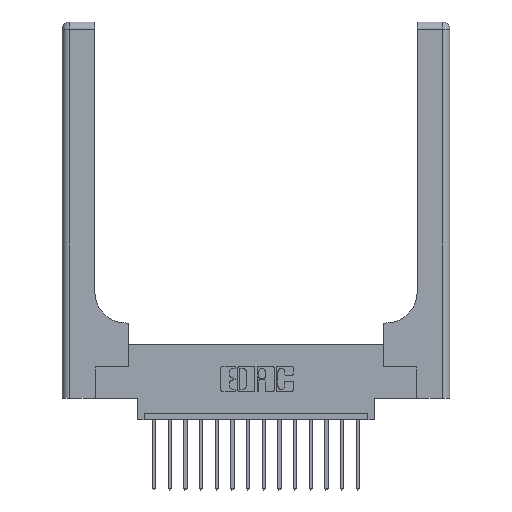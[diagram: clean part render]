
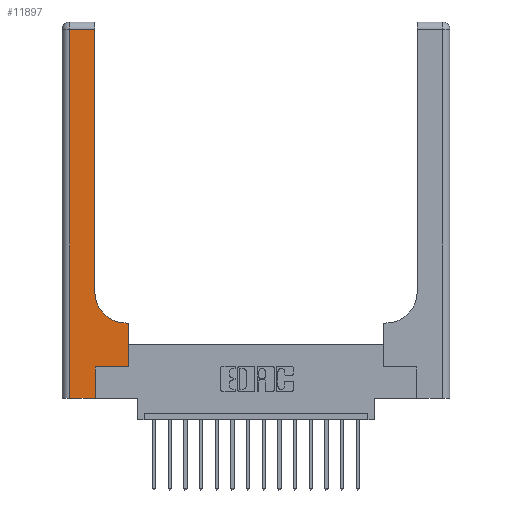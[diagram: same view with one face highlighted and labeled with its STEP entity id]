
A CAD part, top view. The second image highlights one B-rep face of the part: STEP entity #11897.
In plain terms, the highlighted planar face has unit normal (0, 0, 1).
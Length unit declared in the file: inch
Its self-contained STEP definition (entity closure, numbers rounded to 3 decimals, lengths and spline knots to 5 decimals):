
#103 = EDGE_CURVE ( 'NONE', #12529, #12269, #13879, .T. ) ;
#304 = EDGE_CURVE ( 'NONE', #2396, #16840, #3853, .T. ) ;
#818 = EDGE_CURVE ( 'NONE', #12269, #13218, #6470, .T. ) ;
#1005 = ORIENTED_EDGE ( 'NONE', *, *, #304, .T. ) ;
#1039 = DIRECTION ( 'NONE',  ( 1., 0., 0. ) ) ;
#1226 = EDGE_CURVE ( 'NONE', #9002, #12529, #13136, .T. ) ;
#1478 = DIRECTION ( 'NONE',  ( -1., 0., 0. ) ) ;
#1930 = CARTESIAN_POINT ( 'NONE',  ( 0.26, 0.85, 0.37 ) ) ;
#2396 = VERTEX_POINT ( 'NONE', #14128 ) ;
#2476 = VECTOR ( 'NONE', #17531, 39.37008 ) ;
#2568 = EDGE_CURVE ( 'NONE', #16840, #5805, #7296, .T. ) ;
#3481 = ORIENTED_EDGE ( 'NONE', *, *, #103, .T. ) ;
#3629 = CARTESIAN_POINT ( 'NONE',  ( 0.51, 0.85, 0.37 ) ) ;
#3701 = LINE ( 'NONE', #14926, #17962 ) ;
#3853 = CIRCLE ( 'NONE', #5642, 0.25 ) ;
#3968 = ORIENTED_EDGE ( 'NONE', *, *, #2568, .T. ) ;
#4846 = CARTESIAN_POINT ( 'NONE',  ( 0.265, 0.25, 0.37 ) ) ;
#4978 = ORIENTED_EDGE ( 'NONE', *, *, #8151, .T. ) ;
#4997 = PLANE ( 'NONE',  #7004 ) ;
#5442 = CARTESIAN_POINT ( 'NONE',  ( 0.06, 2.94, 0.37 ) ) ;
#5642 = AXIS2_PLACEMENT_3D ( 'NONE', #3629, #17910, #1039 ) ;
#5696 = EDGE_CURVE ( 'NONE', #7643, #2396, #13379, .T. ) ;
#5805 = VERTEX_POINT ( 'NONE', #12971 ) ;
#6012 = DIRECTION ( 'NONE',  ( 0., 0., -1. ) ) ;
#6470 = LINE ( 'NONE', #17800, #13881 ) ;
#6782 = VERTEX_POINT ( 'NONE', #12274 ) ;
#7004 = AXIS2_PLACEMENT_3D ( 'NONE', #10607, #6012, #14834 ) ;
#7296 = LINE ( 'NONE', #15960, #2476 ) ;
#7643 = VERTEX_POINT ( 'NONE', #18095 ) ;
#7826 = DIRECTION ( 'NONE',  ( 0., 1., 0. ) ) ;
#8019 = CARTESIAN_POINT ( 'NONE',  ( 0.528, 0.25, 0.37 ) ) ;
#8151 = EDGE_CURVE ( 'NONE', #6782, #7643, #14922, .T. ) ;
#9002 = VERTEX_POINT ( 'NONE', #5442 ) ;
#9405 = CARTESIAN_POINT ( 'NONE',  ( 0.26, 0.6, 0.37 ) ) ;
#9704 = ORIENTED_EDGE ( 'NONE', *, *, #5696, .T. ) ;
#10588 = CARTESIAN_POINT ( 'NONE',  ( 0.265, 0., 0.37 ) ) ;
#10607 = CARTESIAN_POINT ( 'NONE',  ( 0., 3., 0.37 ) ) ;
#10728 = ORIENTED_EDGE ( 'NONE', *, *, #18039, .T. ) ;
#11309 = DIRECTION ( 'NONE',  ( 1., 0., 0. ) ) ;
#11392 = CARTESIAN_POINT ( 'NONE',  ( 0.265, 0.25, 0.37 ) ) ;
#11540 = VECTOR ( 'NONE', #17174, 39.37008 ) ;
#11724 = ORIENTED_EDGE ( 'NONE', *, *, #818, .T. ) ;
#11817 = EDGE_LOOP ( 'NONE', ( #3968, #12186, #13964, #3481, #11724, #10728, #4978, #9704, #1005 ) ) ;
#11833 = LINE ( 'NONE', #4846, #11540 ) ;
#11897 = ADVANCED_FACE ( 'NONE', ( #16122 ), #4997, .F. ) ;
#12186 = ORIENTED_EDGE ( 'NONE', *, *, #15193, .T. ) ;
#12269 = VERTEX_POINT ( 'NONE', #10588 ) ;
#12274 = CARTESIAN_POINT ( 'NONE',  ( 0.528, 0.25, 0.37 ) ) ;
#12529 = VERTEX_POINT ( 'NONE', #16079 ) ;
#12971 = CARTESIAN_POINT ( 'NONE',  ( 0.26, 2.94, 0.37 ) ) ;
#13136 = LINE ( 'NONE', #16069, #15361 ) ;
#13218 = VERTEX_POINT ( 'NONE', #11392 ) ;
#13379 = LINE ( 'NONE', #9405, #13921 ) ;
#13410 = DIRECTION ( 'NONE',  ( 0., -1., 0. ) ) ;
#13839 = VECTOR ( 'NONE', #11309, 39.37008 ) ;
#13879 = LINE ( 'NONE', #18121, #13839 ) ;
#13881 = VECTOR ( 'NONE', #16326, 39.37008 ) ;
#13921 = VECTOR ( 'NONE', #17696, 39.37008 ) ;
#13964 = ORIENTED_EDGE ( 'NONE', *, *, #1226, .T. ) ;
#14128 = CARTESIAN_POINT ( 'NONE',  ( 0.51, 0.6, 0.37 ) ) ;
#14834 = DIRECTION ( 'NONE',  ( -1., 0., 0. ) ) ;
#14922 = LINE ( 'NONE', #8019, #15232 ) ;
#14926 = CARTESIAN_POINT ( 'NONE',  ( 0., 2.94, 0.37 ) ) ;
#15193 = EDGE_CURVE ( 'NONE', #5805, #9002, #3701, .T. ) ;
#15232 = VECTOR ( 'NONE', #7826, 39.37008 ) ;
#15361 = VECTOR ( 'NONE', #13410, 39.37008 ) ;
#15960 = CARTESIAN_POINT ( 'NONE',  ( 0.26, 3., 0.37 ) ) ;
#16069 = CARTESIAN_POINT ( 'NONE',  ( 0.06, 3., 0.37 ) ) ;
#16079 = CARTESIAN_POINT ( 'NONE',  ( 0.06, 0., 0.37 ) ) ;
#16122 = FACE_OUTER_BOUND ( 'NONE', #11817, .T. ) ;
#16326 = DIRECTION ( 'NONE',  ( 0., 1., 0. ) ) ;
#16840 = VERTEX_POINT ( 'NONE', #1930 ) ;
#17174 = DIRECTION ( 'NONE',  ( 1., 0., 0. ) ) ;
#17531 = DIRECTION ( 'NONE',  ( 0., 1., 0. ) ) ;
#17696 = DIRECTION ( 'NONE',  ( -1., 0., 0. ) ) ;
#17800 = CARTESIAN_POINT ( 'NONE',  ( 0.265, 0., 0.37 ) ) ;
#17910 = DIRECTION ( 'NONE',  ( 0., 0., -1. ) ) ;
#17962 = VECTOR ( 'NONE', #1478, 39.37008 ) ;
#18039 = EDGE_CURVE ( 'NONE', #13218, #6782, #11833, .T. ) ;
#18095 = CARTESIAN_POINT ( 'NONE',  ( 0.528, 0.6, 0.37 ) ) ;
#18121 = CARTESIAN_POINT ( 'NONE',  ( 0., 0., 0.37 ) ) ;
